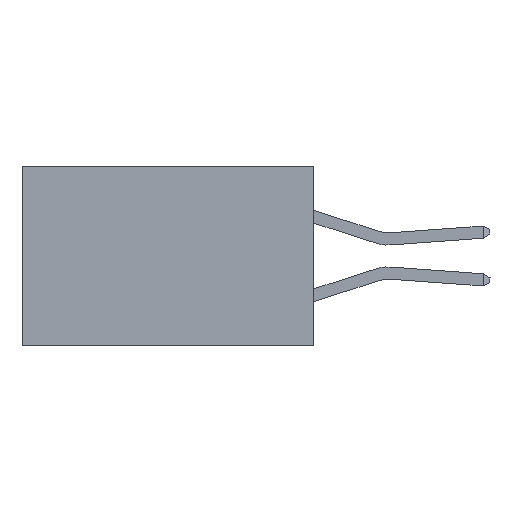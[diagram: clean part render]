
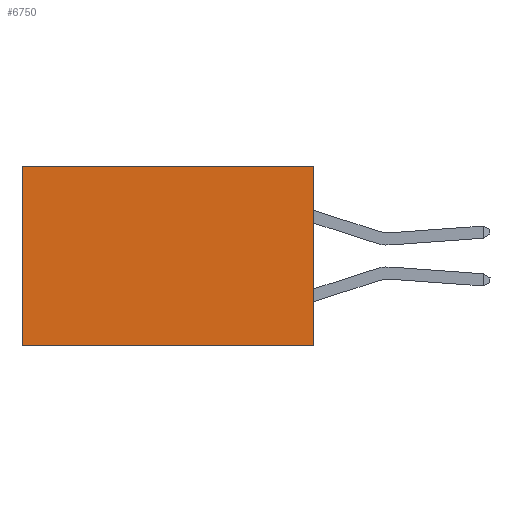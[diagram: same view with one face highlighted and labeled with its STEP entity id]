
A CAD part, left-side view. The second image highlights one B-rep face of the part: STEP entity #6750.
In plain terms, the highlighted planar face has unit normal (-1, 0, 0).
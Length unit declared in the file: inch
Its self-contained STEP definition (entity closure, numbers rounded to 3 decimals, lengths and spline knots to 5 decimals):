
#338 = EDGE_LOOP ( 'NONE', ( #5050, #6030, #5687, #5371 ) ) ;
#858 = EDGE_CURVE ( 'NONE', #904, #11058, #7563, .T. ) ;
#904 = VERTEX_POINT ( 'NONE', #11568 ) ;
#1745 = DIRECTION ( 'NONE',  ( 0., 0., -1. ) ) ;
#1791 = DIRECTION ( 'NONE',  ( 1., 0., 0. ) ) ;
#1802 = PLANE ( 'NONE',  #6526 ) ;
#1815 = LINE ( 'NONE', #6916, #2122 ) ;
#2122 = VECTOR ( 'NONE', #6888, 39.37008 ) ;
#2139 = CARTESIAN_POINT ( 'NONE',  ( 0.2875, 0., 0. ) ) ;
#2632 = VECTOR ( 'NONE', #3373, 39.37008 ) ;
#2790 = VECTOR ( 'NONE', #8289, 39.37008 ) ;
#3373 = DIRECTION ( 'NONE',  ( 0., 1., 0. ) ) ;
#3574 = CARTESIAN_POINT ( 'NONE',  ( 0.2875, 0., 0. ) ) ;
#4143 = VECTOR ( 'NONE', #6918, 39.37008 ) ;
#4177 = EDGE_CURVE ( 'NONE', #11058, #4725, #5230, .T. ) ;
#4725 = VERTEX_POINT ( 'NONE', #5034 ) ;
#5034 = CARTESIAN_POINT ( 'NONE',  ( 0.2875, 0.6, -0.37 ) ) ;
#5050 = ORIENTED_EDGE ( 'NONE', *, *, #4177, .T. ) ;
#5230 = LINE ( 'NONE', #10069, #2790 ) ;
#5371 = ORIENTED_EDGE ( 'NONE', *, *, #858, .T. ) ;
#5687 = ORIENTED_EDGE ( 'NONE', *, *, #7325, .F. ) ;
#5761 = FACE_OUTER_BOUND ( 'NONE', #338, .T. ) ;
#5980 = CARTESIAN_POINT ( 'NONE',  ( 0.2875, 0., -0.37 ) ) ;
#6030 = ORIENTED_EDGE ( 'NONE', *, *, #9560, .F. ) ;
#6526 = AXIS2_PLACEMENT_3D ( 'NONE', #2139, #1791, #1745 ) ;
#6750 = ADVANCED_FACE ( 'NONE', ( #5761 ), #1802, .F. ) ;
#6888 = DIRECTION ( 'NONE',  ( 0., 0., -1. ) ) ;
#6916 = CARTESIAN_POINT ( 'NONE',  ( 0.2875, 0., 0. ) ) ;
#6918 = DIRECTION ( 'NONE',  ( 0., 1., 0. ) ) ;
#7325 = EDGE_CURVE ( 'NONE', #904, #10387, #1815, .T. ) ;
#7563 = LINE ( 'NONE', #3574, #2632 ) ;
#8289 = DIRECTION ( 'NONE',  ( 0., 0., -1. ) ) ;
#9040 = LINE ( 'NONE', #5980, #4143 ) ;
#9560 = EDGE_CURVE ( 'NONE', #10387, #4725, #9040, .T. ) ;
#9711 = CARTESIAN_POINT ( 'NONE',  ( 0.2875, 0.6, 0. ) ) ;
#9880 = CARTESIAN_POINT ( 'NONE',  ( 0.2875, 0., -0.37 ) ) ;
#10069 = CARTESIAN_POINT ( 'NONE',  ( 0.2875, 0.6, 0. ) ) ;
#10387 = VERTEX_POINT ( 'NONE', #9880 ) ;
#11058 = VERTEX_POINT ( 'NONE', #9711 ) ;
#11568 = CARTESIAN_POINT ( 'NONE',  ( 0.2875, 0., 0. ) ) ;
